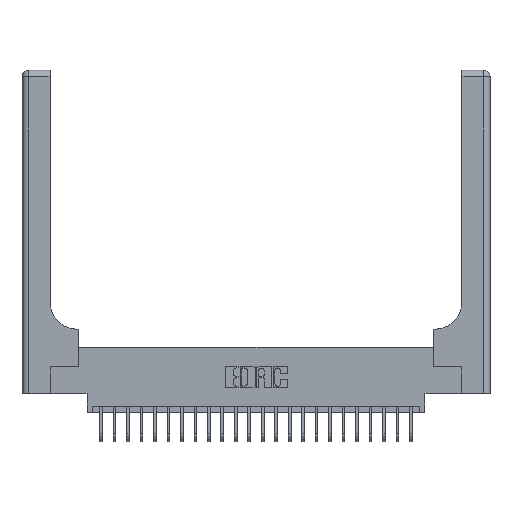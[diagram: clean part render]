
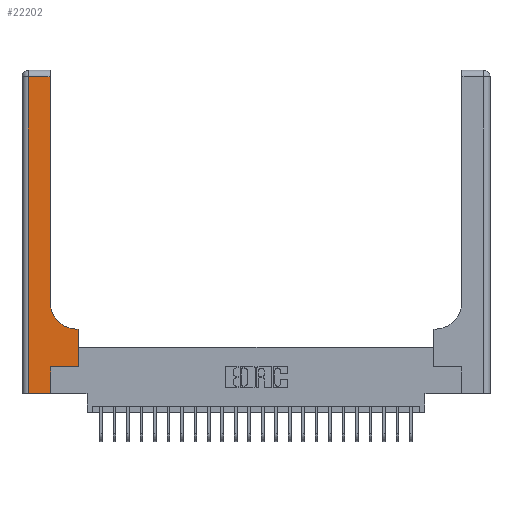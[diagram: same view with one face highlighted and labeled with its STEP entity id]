
A CAD part, top view. The second image highlights one B-rep face of the part: STEP entity #22202.
In plain terms, the highlighted planar face has unit normal (0, 0, 1).
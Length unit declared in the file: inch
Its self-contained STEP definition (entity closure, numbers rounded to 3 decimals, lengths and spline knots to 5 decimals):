
#160 = DIRECTION ( 'NONE',  ( 0., 0., -1. ) ) ;
#294 = DIRECTION ( 'NONE',  ( 1., 0., 0. ) ) ;
#852 = EDGE_CURVE ( 'NONE', #18546, #22014, #15659, .T. ) ;
#1372 = CARTESIAN_POINT ( 'NONE',  ( 0.26, 3., 0.37 ) ) ;
#1689 = ORIENTED_EDGE ( 'NONE', *, *, #852, .T. ) ;
#1895 = AXIS2_PLACEMENT_3D ( 'NONE', #2380, #160, #5674 ) ;
#2380 = CARTESIAN_POINT ( 'NONE',  ( 0., 3., 0.37 ) ) ;
#4079 = ORIENTED_EDGE ( 'NONE', *, *, #12021, .T. ) ;
#4135 = CARTESIAN_POINT ( 'NONE',  ( 0.528, 0.6, 0.37 ) ) ;
#4712 = DIRECTION ( 'NONE',  ( -1., 0., 0. ) ) ;
#4737 = EDGE_LOOP ( 'NONE', ( #4079, #22852, #6191, #1689, #18050, #8780, #8912, #6357, #6597 ) ) ;
#5229 = VERTEX_POINT ( 'NONE', #16845 ) ;
#5261 = AXIS2_PLACEMENT_3D ( 'NONE', #14456, #21858, #294 ) ;
#5674 = DIRECTION ( 'NONE',  ( -1., 0., 0. ) ) ;
#5757 = LINE ( 'NONE', #19937, #14344 ) ;
#6191 = ORIENTED_EDGE ( 'NONE', *, *, #17946, .T. ) ;
#6357 = ORIENTED_EDGE ( 'NONE', *, *, #19767, .T. ) ;
#6597 = ORIENTED_EDGE ( 'NONE', *, *, #7832, .T. ) ;
#6985 = CARTESIAN_POINT ( 'NONE',  ( 0., 2.94, 0.37 ) ) ;
#7361 = VECTOR ( 'NONE', #18259, 39.37008 ) ;
#7585 = VECTOR ( 'NONE', #14304, 39.37008 ) ;
#7599 = LINE ( 'NONE', #9686, #8011 ) ;
#7832 = EDGE_CURVE ( 'NONE', #20557, #13682, #18748, .T. ) ;
#8011 = VECTOR ( 'NONE', #13313, 39.37008 ) ;
#8507 = CARTESIAN_POINT ( 'NONE',  ( 0., 0., 0.37 ) ) ;
#8780 = ORIENTED_EDGE ( 'NONE', *, *, #12863, .T. ) ;
#8912 = ORIENTED_EDGE ( 'NONE', *, *, #14078, .T. ) ;
#9175 = FACE_OUTER_BOUND ( 'NONE', #4737, .T. ) ;
#9186 = VERTEX_POINT ( 'NONE', #18912 ) ;
#9411 = PLANE ( 'NONE',  #1895 ) ;
#9686 = CARTESIAN_POINT ( 'NONE',  ( 0.528, 0.25, 0.37 ) ) ;
#9729 = EDGE_CURVE ( 'NONE', #22014, #14038, #19700, .T. ) ;
#9961 = LINE ( 'NONE', #6985, #19089 ) ;
#12021 = EDGE_CURVE ( 'NONE', #13682, #22116, #15318, .T. ) ;
#12664 = CARTESIAN_POINT ( 'NONE',  ( 0.265, 0., 0.37 ) ) ;
#12863 = EDGE_CURVE ( 'NONE', #14038, #9186, #5757, .T. ) ;
#12965 = LINE ( 'NONE', #16363, #7361 ) ;
#13180 = DIRECTION ( 'NONE',  ( -1., 0., 0. ) ) ;
#13313 = DIRECTION ( 'NONE',  ( 0., 1., 0. ) ) ;
#13682 = VERTEX_POINT ( 'NONE', #19635 ) ;
#14038 = VERTEX_POINT ( 'NONE', #21887 ) ;
#14078 = EDGE_CURVE ( 'NONE', #9186, #14843, #7599, .T. ) ;
#14304 = DIRECTION ( 'NONE',  ( 0., 1., 0. ) ) ;
#14344 = VECTOR ( 'NONE', #14407, 39.37008 ) ;
#14407 = DIRECTION ( 'NONE',  ( 1., 0., 0. ) ) ;
#14456 = CARTESIAN_POINT ( 'NONE',  ( 0.51, 0.85, 0.37 ) ) ;
#14520 = VECTOR ( 'NONE', #4712, 39.37008 ) ;
#14843 = VERTEX_POINT ( 'NONE', #4135 ) ;
#15318 = LINE ( 'NONE', #1372, #20322 ) ;
#15659 = LINE ( 'NONE', #8507, #20415 ) ;
#16363 = CARTESIAN_POINT ( 'NONE',  ( 0.06, 3., 0.37 ) ) ;
#16845 = CARTESIAN_POINT ( 'NONE',  ( 0.06, 2.94, 0.37 ) ) ;
#17946 = EDGE_CURVE ( 'NONE', #5229, #18546, #12965, .T. ) ;
#18050 = ORIENTED_EDGE ( 'NONE', *, *, #9729, .T. ) ;
#18259 = DIRECTION ( 'NONE',  ( 0., -1., 0. ) ) ;
#18546 = VERTEX_POINT ( 'NONE', #19024 ) ;
#18748 = CIRCLE ( 'NONE', #5261, 0.25 ) ;
#18912 = CARTESIAN_POINT ( 'NONE',  ( 0.528, 0.25, 0.37 ) ) ;
#19024 = CARTESIAN_POINT ( 'NONE',  ( 0.06, 0., 0.37 ) ) ;
#19089 = VECTOR ( 'NONE', #13180, 39.37008 ) ;
#19635 = CARTESIAN_POINT ( 'NONE',  ( 0.26, 0.85, 0.37 ) ) ;
#19700 = LINE ( 'NONE', #12664, #7585 ) ;
#19767 = EDGE_CURVE ( 'NONE', #14843, #20557, #22184, .T. ) ;
#19937 = CARTESIAN_POINT ( 'NONE',  ( 0.265, 0.25, 0.37 ) ) ;
#20274 = CARTESIAN_POINT ( 'NONE',  ( 0.51, 0.6, 0.37 ) ) ;
#20322 = VECTOR ( 'NONE', #22463, 39.37008 ) ;
#20415 = VECTOR ( 'NONE', #22798, 39.37008 ) ;
#20557 = VERTEX_POINT ( 'NONE', #20274 ) ;
#21858 = DIRECTION ( 'NONE',  ( 0., 0., -1. ) ) ;
#21882 = EDGE_CURVE ( 'NONE', #22116, #5229, #9961, .T. ) ;
#21887 = CARTESIAN_POINT ( 'NONE',  ( 0.265, 0.25, 0.37 ) ) ;
#22014 = VERTEX_POINT ( 'NONE', #22534 ) ;
#22116 = VERTEX_POINT ( 'NONE', #22991 ) ;
#22184 = LINE ( 'NONE', #22533, #14520 ) ;
#22202 = ADVANCED_FACE ( 'NONE', ( #9175 ), #9411, .F. ) ;
#22463 = DIRECTION ( 'NONE',  ( 0., 1., 0. ) ) ;
#22533 = CARTESIAN_POINT ( 'NONE',  ( 0.26, 0.6, 0.37 ) ) ;
#22534 = CARTESIAN_POINT ( 'NONE',  ( 0.265, 0., 0.37 ) ) ;
#22798 = DIRECTION ( 'NONE',  ( 1., 0., 0. ) ) ;
#22852 = ORIENTED_EDGE ( 'NONE', *, *, #21882, .T. ) ;
#22991 = CARTESIAN_POINT ( 'NONE',  ( 0.26, 2.94, 0.37 ) ) ;
